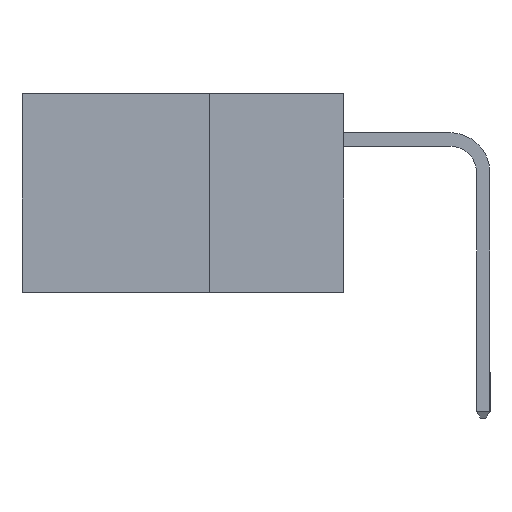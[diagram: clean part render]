
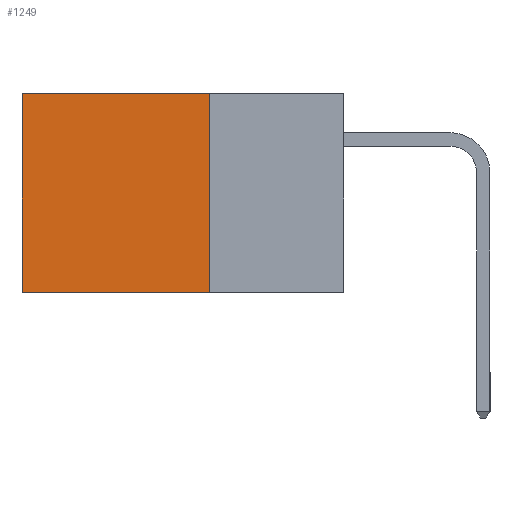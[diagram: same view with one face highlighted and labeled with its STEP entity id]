
A CAD part, left-side view. The second image highlights one B-rep face of the part: STEP entity #1249.
In plain terms, the highlighted planar face has unit normal (-1, 0, 0).
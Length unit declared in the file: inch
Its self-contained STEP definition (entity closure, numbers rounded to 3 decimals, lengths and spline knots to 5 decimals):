
#100 = VERTEX_POINT ( 'NONE', #8761 ) ;
#166 = CARTESIAN_POINT ( 'NONE',  ( 0.2615, 0.6, 0. ) ) ;
#201 = ORIENTED_EDGE ( 'NONE', *, *, #2678, .T. ) ;
#335 = CARTESIAN_POINT ( 'NONE',  ( 0.2615, 0.6, -0.37 ) ) ;
#454 = VECTOR ( 'NONE', #2956, 39.37008 ) ;
#465 = CARTESIAN_POINT ( 'NONE',  ( 0.2615, 0.25, -0.37 ) ) ;
#478 = VECTOR ( 'NONE', #606, 39.37008 ) ;
#515 = LINE ( 'NONE', #4680, #7867 ) ;
#606 = DIRECTION ( 'NONE',  ( 0., 1., 0. ) ) ;
#1079 = EDGE_LOOP ( 'NONE', ( #2005, #8752, #8568, #201 ) ) ;
#1249 = ADVANCED_FACE ( 'NONE', ( #6782 ), #2868, .F. ) ;
#1268 = DIRECTION ( 'NONE',  ( 0., 0., -1. ) ) ;
#1637 = CARTESIAN_POINT ( 'NONE',  ( 0.2615, 0.6, -0.37 ) ) ;
#1840 = VERTEX_POINT ( 'NONE', #166 ) ;
#1949 = CARTESIAN_POINT ( 'NONE',  ( 0.2615, 0.25, -0.37 ) ) ;
#2005 = ORIENTED_EDGE ( 'NONE', *, *, #4534, .T. ) ;
#2317 = VERTEX_POINT ( 'NONE', #1637 ) ;
#2356 = CARTESIAN_POINT ( 'NONE',  ( 0.2615, 0.25, 0. ) ) ;
#2678 = EDGE_CURVE ( 'NONE', #100, #1840, #8405, .T. ) ;
#2868 = PLANE ( 'NONE',  #8518 ) ;
#2956 = DIRECTION ( 'NONE',  ( 0., 1., 0. ) ) ;
#3296 = DIRECTION ( 'NONE',  ( 0., 0., -1. ) ) ;
#3407 = VERTEX_POINT ( 'NONE', #465 ) ;
#3776 = LINE ( 'NONE', #335, #8143 ) ;
#4002 = LINE ( 'NONE', #7530, #478 ) ;
#4202 = DIRECTION ( 'NONE',  ( 1., 0., 0. ) ) ;
#4534 = EDGE_CURVE ( 'NONE', #1840, #2317, #3776, .T. ) ;
#4592 = EDGE_CURVE ( 'NONE', #3407, #2317, #4002, .T. ) ;
#4680 = CARTESIAN_POINT ( 'NONE',  ( 0.2615, 0.25, -0.37 ) ) ;
#5854 = DIRECTION ( 'NONE',  ( 0., 0., -1. ) ) ;
#6600 = EDGE_CURVE ( 'NONE', #100, #3407, #515, .T. ) ;
#6782 = FACE_OUTER_BOUND ( 'NONE', #1079, .T. ) ;
#7530 = CARTESIAN_POINT ( 'NONE',  ( 0.2615, 0.25, -0.37 ) ) ;
#7867 = VECTOR ( 'NONE', #3296, 39.37008 ) ;
#8143 = VECTOR ( 'NONE', #5854, 39.37008 ) ;
#8405 = LINE ( 'NONE', #2356, #454 ) ;
#8518 = AXIS2_PLACEMENT_3D ( 'NONE', #1949, #4202, #1268 ) ;
#8568 = ORIENTED_EDGE ( 'NONE', *, *, #6600, .F. ) ;
#8752 = ORIENTED_EDGE ( 'NONE', *, *, #4592, .F. ) ;
#8761 = CARTESIAN_POINT ( 'NONE',  ( 0.2615, 0.25, 0. ) ) ;
